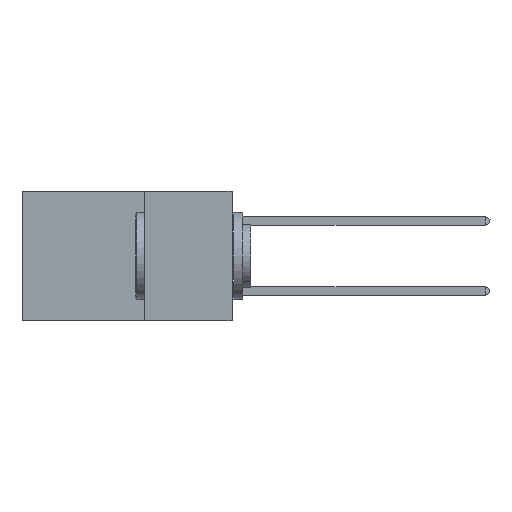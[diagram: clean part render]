
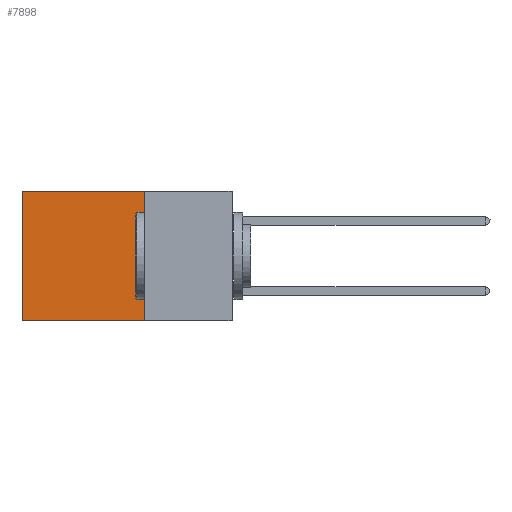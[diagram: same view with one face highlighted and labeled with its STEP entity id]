
A CAD part, left-side view. The second image highlights one B-rep face of the part: STEP entity #7898.
In plain terms, the highlighted planar face has unit normal (-1, 0, 0).
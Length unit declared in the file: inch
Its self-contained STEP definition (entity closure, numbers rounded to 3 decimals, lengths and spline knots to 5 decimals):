
#735 = VERTEX_POINT ( 'NONE', #10211 ) ;
#2840 = DIRECTION ( 'NONE',  ( 0., 1., 0. ) ) ;
#3897 = DIRECTION ( 'NONE',  ( 1., 0., 0. ) ) ;
#4070 = ORIENTED_EDGE ( 'NONE', *, *, #9092, .F. ) ;
#4452 = CARTESIAN_POINT ( 'NONE',  ( 0.2875, 0.6, -0.37 ) ) ;
#7367 = CARTESIAN_POINT ( 'NONE',  ( 0.2875, 0.25, -0.37 ) ) ;
#7898 = ADVANCED_FACE ( 'NONE', ( #23410 ), #29316, .F. ) ;
#8147 = CARTESIAN_POINT ( 'NONE',  ( 0.2875, 0.25, 0. ) ) ;
#9092 = EDGE_CURVE ( 'NONE', #735, #29742, #15676, .T. ) ;
#9686 = CARTESIAN_POINT ( 'NONE',  ( 0.2875, 0.6, 0. ) ) ;
#10211 = CARTESIAN_POINT ( 'NONE',  ( 0.2875, 0.25, 0. ) ) ;
#10611 = CARTESIAN_POINT ( 'NONE',  ( 0.2875, 0.25, 0. ) ) ;
#11215 = EDGE_CURVE ( 'NONE', #29742, #27593, #18329, .T. ) ;
#11708 = DIRECTION ( 'NONE',  ( 0., 1., 0. ) ) ;
#11876 = LINE ( 'NONE', #25689, #13380 ) ;
#12967 = EDGE_CURVE ( 'NONE', #20635, #27593, #29581, .T. ) ;
#13172 = VECTOR ( 'NONE', #2840, 39.37008 ) ;
#13380 = VECTOR ( 'NONE', #11708, 39.37008 ) ;
#14145 = EDGE_CURVE ( 'NONE', #735, #20635, #11876, .T. ) ;
#14273 = CARTESIAN_POINT ( 'NONE',  ( 0.2875, 0.25, -0.37 ) ) ;
#15676 = LINE ( 'NONE', #10611, #24880 ) ;
#17373 = DIRECTION ( 'NONE',  ( 0., 0., -1. ) ) ;
#18329 = LINE ( 'NONE', #14273, #13172 ) ;
#20635 = VERTEX_POINT ( 'NONE', #9686 ) ;
#21789 = ORIENTED_EDGE ( 'NONE', *, *, #14145, .T. ) ;
#22570 = DIRECTION ( 'NONE',  ( 0., 0., -1. ) ) ;
#22734 = AXIS2_PLACEMENT_3D ( 'NONE', #8147, #3897, #22570 ) ;
#23410 = FACE_OUTER_BOUND ( 'NONE', #29591, .T. ) ;
#24880 = VECTOR ( 'NONE', #17373, 39.37008 ) ;
#24894 = DIRECTION ( 'NONE',  ( 0., 0., -1. ) ) ;
#25611 = CARTESIAN_POINT ( 'NONE',  ( 0.2875, 0.6, 0. ) ) ;
#25689 = CARTESIAN_POINT ( 'NONE',  ( 0.2875, 0.25, 0. ) ) ;
#26819 = ORIENTED_EDGE ( 'NONE', *, *, #12967, .T. ) ;
#27018 = ORIENTED_EDGE ( 'NONE', *, *, #11215, .F. ) ;
#27593 = VERTEX_POINT ( 'NONE', #4452 ) ;
#28100 = VECTOR ( 'NONE', #24894, 39.37008 ) ;
#29316 = PLANE ( 'NONE',  #22734 ) ;
#29581 = LINE ( 'NONE', #25611, #28100 ) ;
#29591 = EDGE_LOOP ( 'NONE', ( #26819, #27018, #4070, #21789 ) ) ;
#29742 = VERTEX_POINT ( 'NONE', #7367 ) ;
